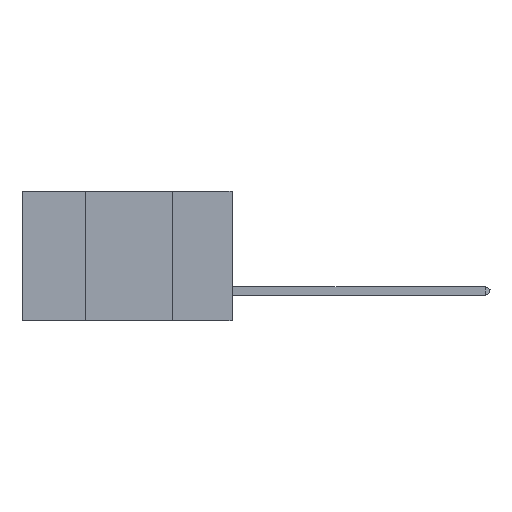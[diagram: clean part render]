
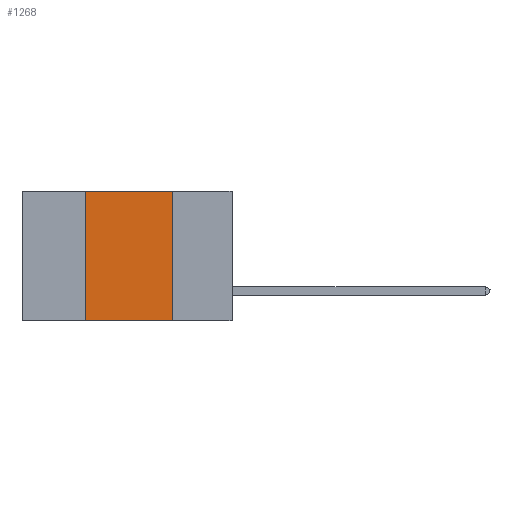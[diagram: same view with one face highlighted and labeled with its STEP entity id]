
A CAD part, left-side view. The second image highlights one B-rep face of the part: STEP entity #1268.
In plain terms, the highlighted planar face has unit normal (-1, 0, 0).
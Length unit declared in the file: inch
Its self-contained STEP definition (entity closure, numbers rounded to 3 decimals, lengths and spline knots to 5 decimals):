
#832 = ORIENTED_EDGE ( 'NONE', *, *, #16635, .F. ) ;
#1268 = ADVANCED_FACE ( 'NONE', ( #19276 ), #30252, .F. ) ;
#1961 = LINE ( 'NONE', #5946, #25324 ) ;
#2764 = EDGE_CURVE ( 'NONE', #28326, #25579, #1961, .T. ) ;
#3462 = VERTEX_POINT ( 'NONE', #25221 ) ;
#4143 = CARTESIAN_POINT ( 'NONE',  ( 0., 0.17, 0. ) ) ;
#4807 = VECTOR ( 'NONE', #4817, 39.37008 ) ;
#4817 = DIRECTION ( 'NONE',  ( 0., 0., 1. ) ) ;
#5225 = LINE ( 'NONE', #20900, #31556 ) ;
#5248 = EDGE_CURVE ( 'NONE', #3462, #14341, #29541, .T. ) ;
#5839 = CARTESIAN_POINT ( 'NONE',  ( 0., 0.6, 0. ) ) ;
#5946 = CARTESIAN_POINT ( 'NONE',  ( 0., 0.6, 0. ) ) ;
#6631 = ORIENTED_EDGE ( 'NONE', *, *, #2764, .F. ) ;
#10168 = EDGE_LOOP ( 'NONE', ( #15458, #6631, #832, #18677 ) ) ;
#14341 = VERTEX_POINT ( 'NONE', #15671 ) ;
#15458 = ORIENTED_EDGE ( 'NONE', *, *, #16294, .F. ) ;
#15636 = DIRECTION ( 'NONE',  ( 0., 0., -1. ) ) ;
#15671 = CARTESIAN_POINT ( 'NONE',  ( 0., 0.17, -0.37 ) ) ;
#15841 = DIRECTION ( 'NONE',  ( 1., 0., 0. ) ) ;
#16294 = EDGE_CURVE ( 'NONE', #25579, #14341, #5225, .T. ) ;
#16517 = DIRECTION ( 'NONE',  ( 0., -1., 0. ) ) ;
#16635 = EDGE_CURVE ( 'NONE', #3462, #28326, #30750, .T. ) ;
#18327 = DIRECTION ( 'NONE',  ( 0., 0., -1. ) ) ;
#18677 = ORIENTED_EDGE ( 'NONE', *, *, #5248, .T. ) ;
#19276 = FACE_OUTER_BOUND ( 'NONE', #10168, .T. ) ;
#19475 = CARTESIAN_POINT ( 'NONE',  ( 0., 0.42, 0. ) ) ;
#20900 = CARTESIAN_POINT ( 'NONE',  ( 0., 0.17, 0. ) ) ;
#22322 = VECTOR ( 'NONE', #16517, 39.37008 ) ;
#22915 = DIRECTION ( 'NONE',  ( 0., -1., 0. ) ) ;
#24692 = AXIS2_PLACEMENT_3D ( 'NONE', #5839, #15841, #15636 ) ;
#25221 = CARTESIAN_POINT ( 'NONE',  ( 0., 0.42, -0.37 ) ) ;
#25324 = VECTOR ( 'NONE', #22915, 39.37008 ) ;
#25579 = VERTEX_POINT ( 'NONE', #4143 ) ;
#25799 = CARTESIAN_POINT ( 'NONE',  ( 0., 0.42, 0. ) ) ;
#28326 = VERTEX_POINT ( 'NONE', #25799 ) ;
#28694 = CARTESIAN_POINT ( 'NONE',  ( 0., 0.6, -0.37 ) ) ;
#29541 = LINE ( 'NONE', #28694, #22322 ) ;
#30252 = PLANE ( 'NONE',  #24692 ) ;
#30750 = LINE ( 'NONE', #19475, #4807 ) ;
#31556 = VECTOR ( 'NONE', #18327, 39.37008 ) ;
